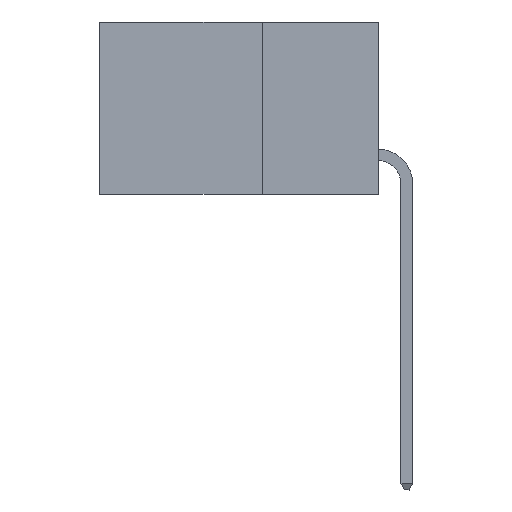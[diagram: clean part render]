
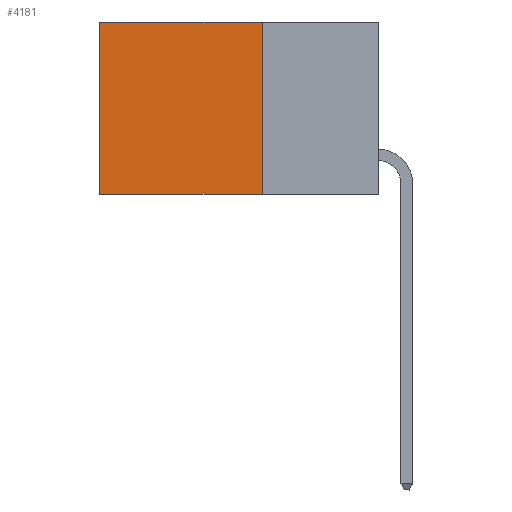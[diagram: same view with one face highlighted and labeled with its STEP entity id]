
A CAD part, left-side view. The second image highlights one B-rep face of the part: STEP entity #4181.
In plain terms, the highlighted planar face has unit normal (-1, 0, 0).
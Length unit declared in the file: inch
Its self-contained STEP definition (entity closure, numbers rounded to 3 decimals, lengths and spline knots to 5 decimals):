
#998 = DIRECTION ( 'NONE',  ( 0., 1., 0. ) ) ;
#1332 = VERTEX_POINT ( 'NONE', #11778 ) ;
#1349 = DIRECTION ( 'NONE',  ( 1., 0., 0. ) ) ;
#3470 = LINE ( 'NONE', #20231, #15201 ) ;
#4030 = DIRECTION ( 'NONE',  ( 0., 0., -1. ) ) ;
#4144 = ORIENTED_EDGE ( 'NONE', *, *, #16384, .T. ) ;
#4181 = ADVANCED_FACE ( 'NONE', ( #13960 ), #20544, .F. ) ;
#4355 = VECTOR ( 'NONE', #19358, 39.37008 ) ;
#5396 = VERTEX_POINT ( 'NONE', #5509 ) ;
#5509 = CARTESIAN_POINT ( 'NONE',  ( 0.298, 0.6, -0.37 ) ) ;
#6699 = DIRECTION ( 'NONE',  ( 0., 0., -1. ) ) ;
#7586 = ORIENTED_EDGE ( 'NONE', *, *, #15000, .T. ) ;
#7973 = ORIENTED_EDGE ( 'NONE', *, *, #18517, .F. ) ;
#8182 = LINE ( 'NONE', #19352, #11853 ) ;
#8685 = LINE ( 'NONE', #14614, #4355 ) ;
#10040 = ORIENTED_EDGE ( 'NONE', *, *, #10480, .F. ) ;
#10480 = EDGE_CURVE ( 'NONE', #20311, #10663, #8182, .T. ) ;
#10663 = VERTEX_POINT ( 'NONE', #15013 ) ;
#11080 = CARTESIAN_POINT ( 'NONE',  ( 0.298, 0.25, 0. ) ) ;
#11554 = LINE ( 'NONE', #11992, #13760 ) ;
#11778 = CARTESIAN_POINT ( 'NONE',  ( 0.298, 0.6, 0. ) ) ;
#11853 = VECTOR ( 'NONE', #6699, 39.37008 ) ;
#11992 = CARTESIAN_POINT ( 'NONE',  ( 0.298, 0.6, 0. ) ) ;
#12665 = DIRECTION ( 'NONE',  ( 0., 0., -1. ) ) ;
#12867 = CARTESIAN_POINT ( 'NONE',  ( 0.298, 0.25, 0. ) ) ;
#13760 = VECTOR ( 'NONE', #4030, 39.37008 ) ;
#13960 = FACE_OUTER_BOUND ( 'NONE', #18172, .T. ) ;
#14345 = AXIS2_PLACEMENT_3D ( 'NONE', #11080, #1349, #12665 ) ;
#14614 = CARTESIAN_POINT ( 'NONE',  ( 0.298, 0.25, -0.37 ) ) ;
#15000 = EDGE_CURVE ( 'NONE', #1332, #5396, #11554, .T. ) ;
#15013 = CARTESIAN_POINT ( 'NONE',  ( 0.298, 0.25, -0.37 ) ) ;
#15201 = VECTOR ( 'NONE', #998, 39.37008 ) ;
#16384 = EDGE_CURVE ( 'NONE', #20311, #1332, #3470, .T. ) ;
#18172 = EDGE_LOOP ( 'NONE', ( #7586, #7973, #10040, #4144 ) ) ;
#18517 = EDGE_CURVE ( 'NONE', #10663, #5396, #8685, .T. ) ;
#19352 = CARTESIAN_POINT ( 'NONE',  ( 0.298, 0.25, 0. ) ) ;
#19358 = DIRECTION ( 'NONE',  ( 0., 1., 0. ) ) ;
#20231 = CARTESIAN_POINT ( 'NONE',  ( 0.298, 0.25, 0. ) ) ;
#20311 = VERTEX_POINT ( 'NONE', #12867 ) ;
#20544 = PLANE ( 'NONE',  #14345 ) ;
